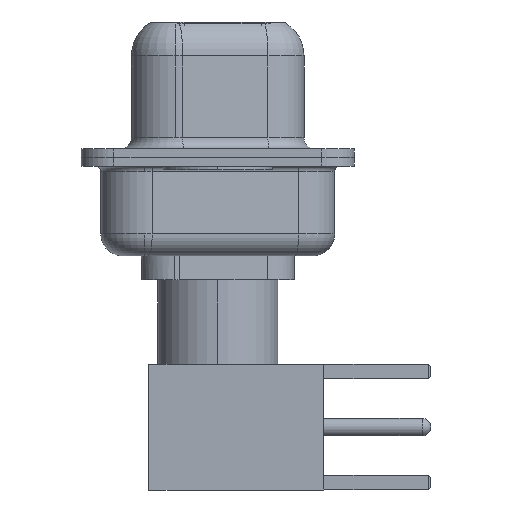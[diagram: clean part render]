
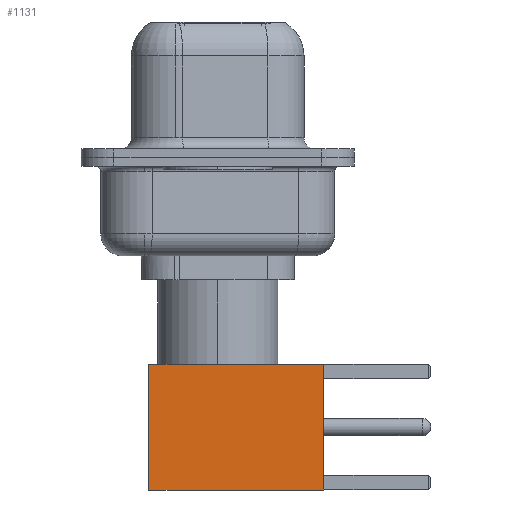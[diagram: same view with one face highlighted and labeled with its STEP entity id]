
A CAD part, left-side view. The second image highlights one B-rep face of the part: STEP entity #1131.
In plain terms, the highlighted face is planar.
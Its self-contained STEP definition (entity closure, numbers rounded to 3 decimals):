
#1131 = ADVANCED_FACE ( 'NONE', ( #4747 ), #16991, .T. ) ;
#1608 = VECTOR ( 'NONE', #4971, 1000. ) ;
#1923 = DIRECTION ( 'NONE',  ( -1., 0., 0. ) ) ;
#2415 = ORIENTED_EDGE ( 'NONE', *, *, #9450, .F. ) ;
#2460 = EDGE_CURVE ( 'NONE', #9310, #3608, #3418, .T. ) ;
#2571 = CARTESIAN_POINT ( 'NONE',  ( -2.875, 2.875, 8. ) ) ;
#3418 = LINE ( 'NONE', #15151, #17194 ) ;
#3538 = CARTESIAN_POINT ( 'NONE',  ( 2.875, 2.875, 8. ) ) ;
#3608 = VERTEX_POINT ( 'NONE', #2571 ) ;
#3803 = DIRECTION ( 'NONE',  ( 0., 0., -1. ) ) ;
#4060 = EDGE_CURVE ( 'NONE', #9310, #8046, #12323, .T. ) ;
#4747 = FACE_OUTER_BOUND ( 'NONE', #8257, .T. ) ;
#4832 = CARTESIAN_POINT ( 'NONE',  ( 2.875, 2.875, 0. ) ) ;
#4971 = DIRECTION ( 'NONE',  ( -1., 0., 0. ) ) ;
#5624 = CARTESIAN_POINT ( 'NONE',  ( 2.875, 2.875, 0. ) ) ;
#6297 = ORIENTED_EDGE ( 'NONE', *, *, #4060, .T. ) ;
#6381 = VECTOR ( 'NONE', #3803, 1000. ) ;
#6452 = DIRECTION ( 'NONE',  ( 0., 0., -1. ) ) ;
#7567 = DIRECTION ( 'NONE',  ( 0., 0., 1. ) ) ;
#7926 = CARTESIAN_POINT ( 'NONE',  ( 2.875, 2.875, 0. ) ) ;
#8046 = VERTEX_POINT ( 'NONE', #5624 ) ;
#8257 = EDGE_LOOP ( 'NONE', ( #6297, #12793, #2415, #10680 ) ) ;
#8778 = AXIS2_PLACEMENT_3D ( 'NONE', #4832, #17090, #7567 ) ;
#9018 = LINE ( 'NONE', #17039, #1608 ) ;
#9039 = VECTOR ( 'NONE', #6452, 1000. ) ;
#9310 = VERTEX_POINT ( 'NONE', #3538 ) ;
#9450 = EDGE_CURVE ( 'NONE', #3608, #11827, #15611, .T. ) ;
#10680 = ORIENTED_EDGE ( 'NONE', *, *, #2460, .F. ) ;
#11827 = VERTEX_POINT ( 'NONE', #15622 ) ;
#11849 = EDGE_CURVE ( 'NONE', #8046, #11827, #9018, .T. ) ;
#12323 = LINE ( 'NONE', #7926, #9039 ) ;
#12793 = ORIENTED_EDGE ( 'NONE', *, *, #11849, .T. ) ;
#15151 = CARTESIAN_POINT ( 'NONE',  ( 0., 2.875, 8. ) ) ;
#15611 = LINE ( 'NONE', #15961, #6381 ) ;
#15622 = CARTESIAN_POINT ( 'NONE',  ( -2.875, 2.875, 0. ) ) ;
#15961 = CARTESIAN_POINT ( 'NONE',  ( -2.875, 2.875, 0. ) ) ;
#16991 = PLANE ( 'NONE',  #8778 ) ;
#17039 = CARTESIAN_POINT ( 'NONE',  ( 0., 2.875, 0. ) ) ;
#17090 = DIRECTION ( 'NONE',  ( 0., 1., 0. ) ) ;
#17194 = VECTOR ( 'NONE', #1923, 1000. ) ;
